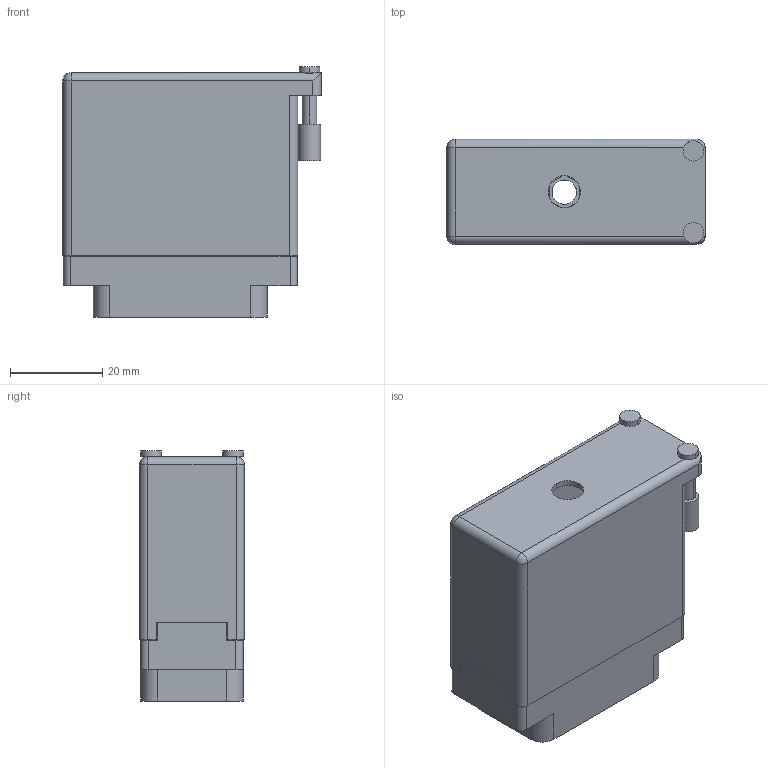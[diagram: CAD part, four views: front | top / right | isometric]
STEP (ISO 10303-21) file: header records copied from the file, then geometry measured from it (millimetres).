
FILE_DESCRIPTION (( 'STEP AP203' ), '1' );
FILE_NAME ('516-038-500-350.STEP', '2020-03-09T20:05:12', ( '' ), ( '' ), 'SwSTEP 2.0', 'SolidWorks 2016', '' );
FILE_SCHEMA (( 'CONFIG_CONTROL_DESIGN' ));
Length unit declared in the file: inch
Products named in the file (4): 516 Plug Insulator_038; 516-230-001_Metal - 038 Side Entry; 516-038-500-350; 516-292-001_500 Contact
Assembly tree (40 placements, depth 2):
  516-038-500-350
    516 Plug Insulator_038
    516-292-001_500 Contact  x38
    516-230-001_Metal - 038 Side Entry
Bounding box: 56.08 x 22.83 x 54.31 mm (x, y, z)
Volume: 18834.9 mm3; surface area: 31869.5 mm2
Topology: 40 solids, 40 shells, 3836 faces, 11127 edges, 7386 vertices
Faces by surface type: plane 2308, cylinder 1296, bspline 228, cone 2, sphere 2
Entity records: 35866 total; most frequent: CARTESIAN_POINT 6362, ORIENTED_EDGE 5970, DIRECTION 5803, EDGE_CURVE 2985, LINE 2211, VECTOR 2211, VERTEX_POINT 1984, AXIS2_PLACEMENT_3D 1796
